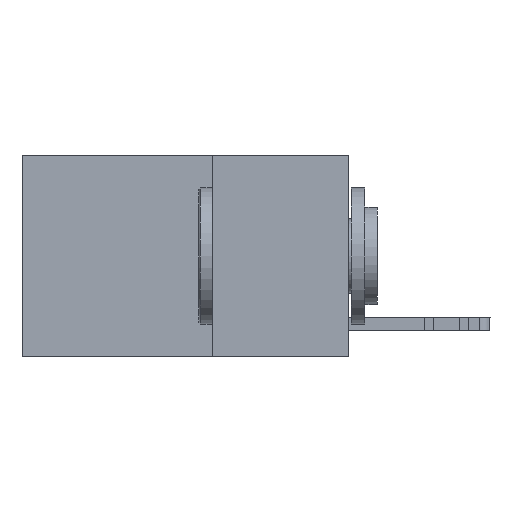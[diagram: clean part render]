
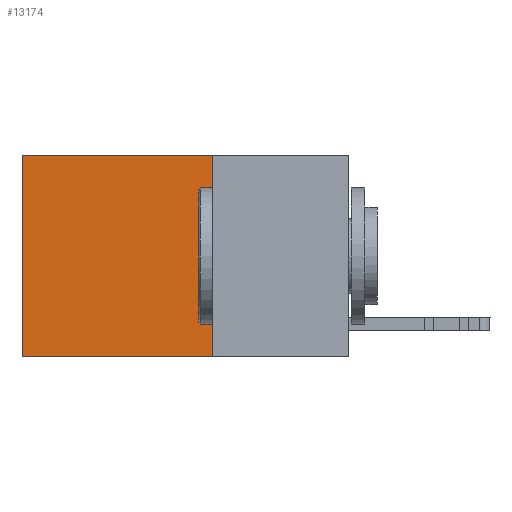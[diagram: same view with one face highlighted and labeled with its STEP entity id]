
A CAD part, left-side view. The second image highlights one B-rep face of the part: STEP entity #13174.
In plain terms, the highlighted planar face has unit normal (-1, 0, 0).
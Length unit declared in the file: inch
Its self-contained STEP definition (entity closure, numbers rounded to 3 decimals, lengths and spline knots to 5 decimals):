
#1248 = EDGE_CURVE ( 'NONE', #11053, #2072, #17633, .T. ) ;
#2072 = VERTEX_POINT ( 'NONE', #22279 ) ;
#2689 = CARTESIAN_POINT ( 'NONE',  ( 0.2625, 0.25, 0. ) ) ;
#3838 = DIRECTION ( 'NONE',  ( 1., 0., 0. ) ) ;
#4736 = ORIENTED_EDGE ( 'NONE', *, *, #17780, .F. ) ;
#4893 = VECTOR ( 'NONE', #13468, 39.37008 ) ;
#6690 = CARTESIAN_POINT ( 'NONE',  ( 0.2625, 0.25, 0. ) ) ;
#6898 = VECTOR ( 'NONE', #9449, 39.37008 ) ;
#7126 = EDGE_LOOP ( 'NONE', ( #16457, #17111, #4736, #7943 ) ) ;
#7580 = LINE ( 'NONE', #2689, #6898 ) ;
#7943 = ORIENTED_EDGE ( 'NONE', *, *, #16947, .T. ) ;
#8842 = CARTESIAN_POINT ( 'NONE',  ( 0.2625, 0.6, 0. ) ) ;
#9331 = PLANE ( 'NONE',  #10885 ) ;
#9449 = DIRECTION ( 'NONE',  ( 0., 0., -1. ) ) ;
#10495 = EDGE_CURVE ( 'NONE', #11004, #2072, #27621, .T. ) ;
#10885 = AXIS2_PLACEMENT_3D ( 'NONE', #18072, #3838, #19319 ) ;
#11004 = VERTEX_POINT ( 'NONE', #8842 ) ;
#11053 = VERTEX_POINT ( 'NONE', #24371 ) ;
#11126 = VECTOR ( 'NONE', #15176, 39.37008 ) ;
#12990 = CARTESIAN_POINT ( 'NONE',  ( 0.2625, 0.25, -0.37 ) ) ;
#13174 = ADVANCED_FACE ( 'NONE', ( #22769 ), #9331, .F. ) ;
#13468 = DIRECTION ( 'NONE',  ( 0., 0., -1. ) ) ;
#15176 = DIRECTION ( 'NONE',  ( 0., 1., 0. ) ) ;
#16457 = ORIENTED_EDGE ( 'NONE', *, *, #10495, .T. ) ;
#16947 = EDGE_CURVE ( 'NONE', #19474, #11004, #18662, .T. ) ;
#17111 = ORIENTED_EDGE ( 'NONE', *, *, #1248, .F. ) ;
#17583 = CARTESIAN_POINT ( 'NONE',  ( 0.2625, 0.25, 0. ) ) ;
#17633 = LINE ( 'NONE', #12990, #11126 ) ;
#17780 = EDGE_CURVE ( 'NONE', #19474, #11053, #7580, .T. ) ;
#17984 = VECTOR ( 'NONE', #19804, 39.37008 ) ;
#18072 = CARTESIAN_POINT ( 'NONE',  ( 0.2625, 0.25, 0. ) ) ;
#18662 = LINE ( 'NONE', #17583, #17984 ) ;
#19319 = DIRECTION ( 'NONE',  ( 0., 0., -1. ) ) ;
#19474 = VERTEX_POINT ( 'NONE', #6690 ) ;
#19804 = DIRECTION ( 'NONE',  ( 0., 1., 0. ) ) ;
#22279 = CARTESIAN_POINT ( 'NONE',  ( 0.2625, 0.6, -0.37 ) ) ;
#22769 = FACE_OUTER_BOUND ( 'NONE', #7126, .T. ) ;
#24371 = CARTESIAN_POINT ( 'NONE',  ( 0.2625, 0.25, -0.37 ) ) ;
#26543 = CARTESIAN_POINT ( 'NONE',  ( 0.2625, 0.6, 0. ) ) ;
#27621 = LINE ( 'NONE', #26543, #4893 ) ;
